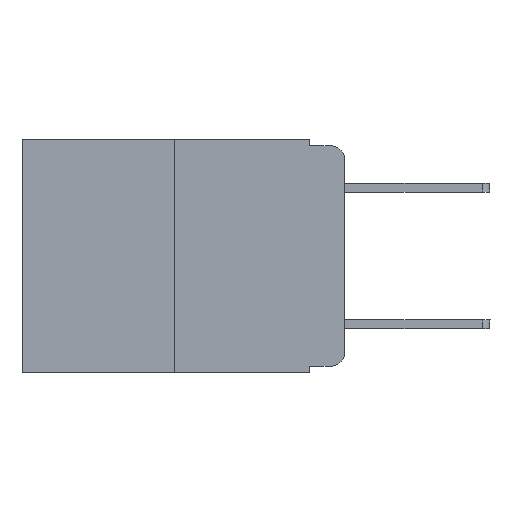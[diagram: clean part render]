
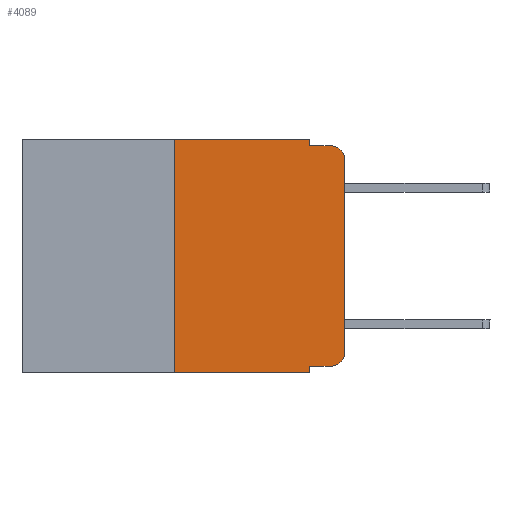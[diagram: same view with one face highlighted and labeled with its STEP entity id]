
A CAD part, left-side view. The second image highlights one B-rep face of the part: STEP entity #4089.
In plain terms, the highlighted planar face has unit normal (-1, 0, 0).
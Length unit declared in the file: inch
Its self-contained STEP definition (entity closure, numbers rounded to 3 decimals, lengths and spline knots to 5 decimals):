
#324 = CARTESIAN_POINT ( 'NONE',  ( 0., 0.051, -0.333 ) ) ;
#334 = VERTEX_POINT ( 'NONE', #3301 ) ;
#609 = CARTESIAN_POINT ( 'NONE',  ( 0., 0., -0.03 ) ) ;
#738 = LINE ( 'NONE', #2335, #8950 ) ;
#826 = VECTOR ( 'NONE', #4500, 39.37008 ) ;
#950 = VERTEX_POINT ( 'NONE', #1815 ) ;
#1145 = CARTESIAN_POINT ( 'NONE',  ( 0., 0.051, -0.01 ) ) ;
#1212 = DIRECTION ( 'NONE',  ( 0., -1., 0. ) ) ;
#1397 = AXIS2_PLACEMENT_3D ( 'NONE', #4045, #1453, #9970 ) ;
#1453 = DIRECTION ( 'NONE',  ( -1., 0., 0. ) ) ;
#1707 = FACE_OUTER_BOUND ( 'NONE', #6381, .T. ) ;
#1725 = EDGE_CURVE ( 'NONE', #950, #5436, #8227, .T. ) ;
#1815 = CARTESIAN_POINT ( 'NONE',  ( 0., 0.02, -0.333 ) ) ;
#2013 = DIRECTION ( 'NONE',  ( 0., 0., -1. ) ) ;
#2050 = VERTEX_POINT ( 'NONE', #6967 ) ;
#2101 = EDGE_CURVE ( 'NONE', #334, #2050, #6191, .T. ) ;
#2331 = ORIENTED_EDGE ( 'NONE', *, *, #10853, .T. ) ;
#2335 = CARTESIAN_POINT ( 'NONE',  ( 0., 0., 0. ) ) ;
#2453 = CIRCLE ( 'NONE', #1397, 0.02 ) ;
#2496 = CARTESIAN_POINT ( 'NONE',  ( 0., 0.473, -0.343 ) ) ;
#2631 = CARTESIAN_POINT ( 'NONE',  ( 0., 0.473, 0. ) ) ;
#3037 = LINE ( 'NONE', #10665, #8929 ) ;
#3117 = DIRECTION ( 'NONE',  ( 0., 0., -1. ) ) ;
#3124 = VERTEX_POINT ( 'NONE', #10652 ) ;
#3301 = CARTESIAN_POINT ( 'NONE',  ( 0., 0.051, 0. ) ) ;
#3474 = DIRECTION ( 'NONE',  ( 0., 0., -1. ) ) ;
#3594 = VERTEX_POINT ( 'NONE', #5579 ) ;
#3636 = AXIS2_PLACEMENT_3D ( 'NONE', #5183, #4124, #3474 ) ;
#3785 = CARTESIAN_POINT ( 'NONE',  ( 0., 0.051, -0.333 ) ) ;
#4000 = EDGE_CURVE ( 'NONE', #3594, #5195, #3037, .T. ) ;
#4045 = CARTESIAN_POINT ( 'NONE',  ( 0., 0.02, -0.03 ) ) ;
#4089 = ADVANCED_FACE ( 'NONE', ( #1707 ), #6781, .F. ) ;
#4091 = DIRECTION ( 'NONE',  ( 0., 0., -1. ) ) ;
#4124 = DIRECTION ( 'NONE',  ( 1., 0., 0. ) ) ;
#4255 = ORIENTED_EDGE ( 'NONE', *, *, #4366, .F. ) ;
#4335 = VECTOR ( 'NONE', #1212, 39.37008 ) ;
#4341 = EDGE_CURVE ( 'NONE', #10142, #950, #10336, .T. ) ;
#4366 = EDGE_CURVE ( 'NONE', #10142, #3124, #6423, .T. ) ;
#4500 = DIRECTION ( 'NONE',  ( 0., -1., 0. ) ) ;
#4790 = EDGE_CURVE ( 'NONE', #2050, #6892, #7830, .T. ) ;
#4862 = AXIS2_PLACEMENT_3D ( 'NONE', #6324, #9906, #4091 ) ;
#4880 = ORIENTED_EDGE ( 'NONE', *, *, #2101, .F. ) ;
#5030 = EDGE_CURVE ( 'NONE', #5436, #5420, #738, .T. ) ;
#5183 = CARTESIAN_POINT ( 'NONE',  ( 0., 0.473, 0. ) ) ;
#5195 = VERTEX_POINT ( 'NONE', #9527 ) ;
#5369 = VECTOR ( 'NONE', #2013, 39.37008 ) ;
#5420 = VERTEX_POINT ( 'NONE', #609 ) ;
#5436 = VERTEX_POINT ( 'NONE', #8238 ) ;
#5579 = CARTESIAN_POINT ( 'NONE',  ( 0., 0.25, -0.343 ) ) ;
#5662 = DIRECTION ( 'NONE',  ( 0., 0., 1. ) ) ;
#5994 = DIRECTION ( 'NONE',  ( 0., -1., 0. ) ) ;
#6191 = LINE ( 'NONE', #9582, #5369 ) ;
#6324 = CARTESIAN_POINT ( 'NONE',  ( 0., 0.02, -0.313 ) ) ;
#6381 = EDGE_LOOP ( 'NONE', ( #7425, #6689, #9222, #4880, #7715, #9902, #2331, #4255, #10925, #8297 ) ) ;
#6423 = LINE ( 'NONE', #8267, #9462 ) ;
#6685 = VECTOR ( 'NONE', #5994, 39.37008 ) ;
#6689 = ORIENTED_EDGE ( 'NONE', *, *, #9294, .T. ) ;
#6781 = PLANE ( 'NONE',  #3636 ) ;
#6892 = VERTEX_POINT ( 'NONE', #8527 ) ;
#6939 = LINE ( 'NONE', #2631, #6685 ) ;
#6967 = CARTESIAN_POINT ( 'NONE',  ( 0., 0.051, -0.01 ) ) ;
#7425 = ORIENTED_EDGE ( 'NONE', *, *, #5030, .T. ) ;
#7715 = ORIENTED_EDGE ( 'NONE', *, *, #8956, .F. ) ;
#7830 = LINE ( 'NONE', #1145, #826 ) ;
#8227 = CIRCLE ( 'NONE', #4862, 0.02 ) ;
#8238 = CARTESIAN_POINT ( 'NONE',  ( 0., 0., -0.313 ) ) ;
#8267 = CARTESIAN_POINT ( 'NONE',  ( 0., 0.051, 0. ) ) ;
#8297 = ORIENTED_EDGE ( 'NONE', *, *, #1725, .T. ) ;
#8527 = CARTESIAN_POINT ( 'NONE',  ( 0., 0.02, -0.01 ) ) ;
#8689 = VECTOR ( 'NONE', #9237, 39.37008 ) ;
#8929 = VECTOR ( 'NONE', #5662, 39.37008 ) ;
#8950 = VECTOR ( 'NONE', #10912, 39.37008 ) ;
#8956 = EDGE_CURVE ( 'NONE', #5195, #334, #6939, .T. ) ;
#9222 = ORIENTED_EDGE ( 'NONE', *, *, #4790, .F. ) ;
#9237 = DIRECTION ( 'NONE',  ( 0., -1., 0. ) ) ;
#9294 = EDGE_CURVE ( 'NONE', #5420, #6892, #2453, .T. ) ;
#9462 = VECTOR ( 'NONE', #3117, 39.37008 ) ;
#9527 = CARTESIAN_POINT ( 'NONE',  ( 0., 0.25, 0. ) ) ;
#9582 = CARTESIAN_POINT ( 'NONE',  ( 0., 0.051, 0. ) ) ;
#9902 = ORIENTED_EDGE ( 'NONE', *, *, #4000, .F. ) ;
#9906 = DIRECTION ( 'NONE',  ( -1., 0., 0. ) ) ;
#9970 = DIRECTION ( 'NONE',  ( 0., 0., -1. ) ) ;
#10142 = VERTEX_POINT ( 'NONE', #3785 ) ;
#10336 = LINE ( 'NONE', #324, #4335 ) ;
#10652 = CARTESIAN_POINT ( 'NONE',  ( 0., 0.051, -0.343 ) ) ;
#10665 = CARTESIAN_POINT ( 'NONE',  ( 0., 0.25, 0. ) ) ;
#10853 = EDGE_CURVE ( 'NONE', #3594, #3124, #10901, .T. ) ;
#10901 = LINE ( 'NONE', #2496, #8689 ) ;
#10912 = DIRECTION ( 'NONE',  ( 0., 0., 1. ) ) ;
#10925 = ORIENTED_EDGE ( 'NONE', *, *, #4341, .T. ) ;
